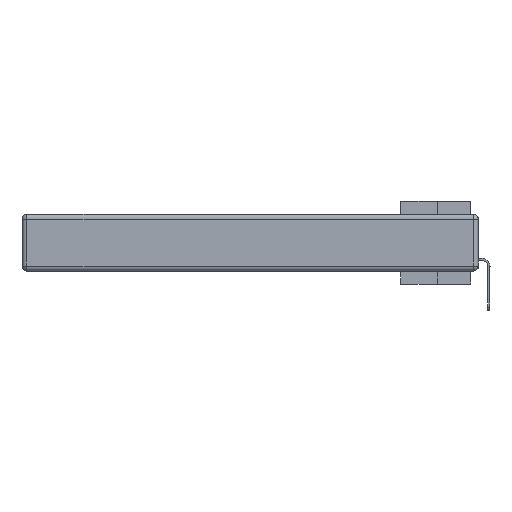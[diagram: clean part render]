
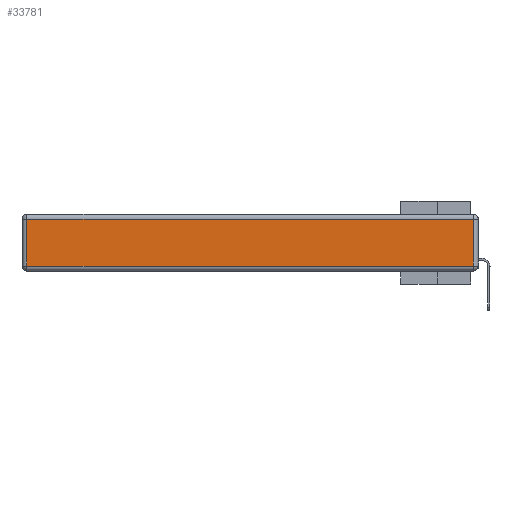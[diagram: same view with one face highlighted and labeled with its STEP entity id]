
A CAD part, left-side view. The second image highlights one B-rep face of the part: STEP entity #33781.
In plain terms, the highlighted planar face has unit normal (-1, 0, 0).
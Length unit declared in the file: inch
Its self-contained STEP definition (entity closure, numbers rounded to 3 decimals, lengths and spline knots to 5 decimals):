
#412 = CARTESIAN_POINT ( 'NONE',  ( 0., 2.72, -0.03 ) ) ;
#594 = VECTOR ( 'NONE', #9508, 39.37008 ) ;
#2215 = ORIENTED_EDGE ( 'NONE', *, *, #26105, .T. ) ;
#3457 = DIRECTION ( 'NONE',  ( 0., -1., 0. ) ) ;
#4194 = EDGE_CURVE ( 'NONE', #24640, #37062, #15662, .T. ) ;
#4912 = ORIENTED_EDGE ( 'NONE', *, *, #4194, .T. ) ;
#8599 = ORIENTED_EDGE ( 'NONE', *, *, #33763, .T. ) ;
#8935 = LINE ( 'NONE', #15685, #594 ) ;
#9246 = CARTESIAN_POINT ( 'NONE',  ( 0., 0., -0.313 ) ) ;
#9479 = CARTESIAN_POINT ( 'NONE',  ( 0., 0.03, -0.343 ) ) ;
#9508 = DIRECTION ( 'NONE',  ( 0., 0., -1. ) ) ;
#9879 = CARTESIAN_POINT ( 'NONE',  ( 0., 2.72, -0.313 ) ) ;
#10982 = VECTOR ( 'NONE', #3457, 39.37008 ) ;
#12146 = LINE ( 'NONE', #9246, #10982 ) ;
#12405 = DIRECTION ( 'NONE',  ( 0., 0., 1. ) ) ;
#15337 = VERTEX_POINT ( 'NONE', #412 ) ;
#15488 = DIRECTION ( 'NONE',  ( -1., 0., 0. ) ) ;
#15662 = LINE ( 'NONE', #9479, #18110 ) ;
#15685 = CARTESIAN_POINT ( 'NONE',  ( 0., 2.72, -0.343 ) ) ;
#18110 = VECTOR ( 'NONE', #36275, 39.37008 ) ;
#18575 = LINE ( 'NONE', #24906, #29789 ) ;
#20840 = EDGE_LOOP ( 'NONE', ( #22392, #4912, #8599, #2215 ) ) ;
#22392 = ORIENTED_EDGE ( 'NONE', *, *, #24102, .T. ) ;
#24102 = EDGE_CURVE ( 'NONE', #33756, #24640, #12146, .T. ) ;
#24640 = VERTEX_POINT ( 'NONE', #27304 ) ;
#24906 = CARTESIAN_POINT ( 'NONE',  ( 0., 2.75, -0.03 ) ) ;
#26105 = EDGE_CURVE ( 'NONE', #15337, #33756, #8935, .T. ) ;
#27304 = CARTESIAN_POINT ( 'NONE',  ( 0., 0.03, -0.313 ) ) ;
#29789 = VECTOR ( 'NONE', #36690, 39.37008 ) ;
#30533 = PLANE ( 'NONE',  #36559 ) ;
#32968 = CARTESIAN_POINT ( 'NONE',  ( 0., 0.03, -0.03 ) ) ;
#33031 = CARTESIAN_POINT ( 'NONE',  ( 0., 0., -0.343 ) ) ;
#33756 = VERTEX_POINT ( 'NONE', #9879 ) ;
#33763 = EDGE_CURVE ( 'NONE', #37062, #15337, #18575, .T. ) ;
#33781 = ADVANCED_FACE ( 'NONE', ( #36119 ), #30533, .T. ) ;
#36119 = FACE_OUTER_BOUND ( 'NONE', #20840, .T. ) ;
#36275 = DIRECTION ( 'NONE',  ( 0., 0., 1. ) ) ;
#36559 = AXIS2_PLACEMENT_3D ( 'NONE', #33031, #15488, #12405 ) ;
#36690 = DIRECTION ( 'NONE',  ( 0., 1., 0. ) ) ;
#37062 = VERTEX_POINT ( 'NONE', #32968 ) ;
